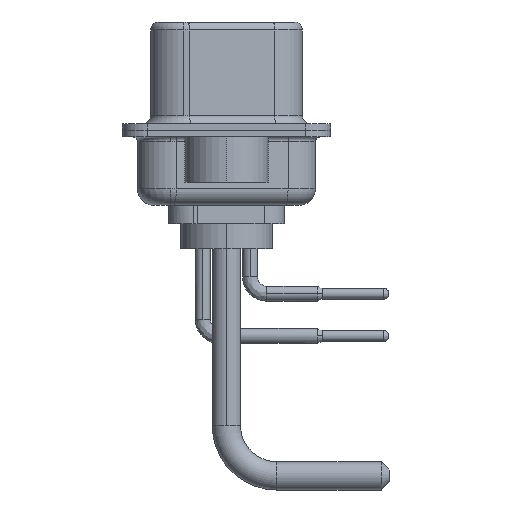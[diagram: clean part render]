
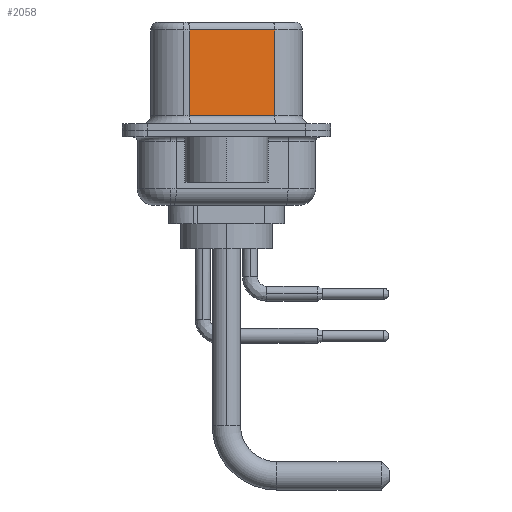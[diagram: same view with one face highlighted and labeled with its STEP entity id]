
A CAD part, left-side view. The second image highlights one B-rep face of the part: STEP entity #2058.
In plain terms, the highlighted planar face has unit normal (-0.985, -0.174, 0).
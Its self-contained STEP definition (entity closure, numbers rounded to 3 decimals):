
#1162 = ORIENTED_EDGE ( 'NONE', *, *, #23147, .F. ) ;
#2058 = ADVANCED_FACE ( 'NONE', ( #18580 ), #20807, .F. ) ;
#2570 = DIRECTION ( 'NONE',  ( 0.174, -0.985, 0. ) ) ;
#2748 = VERTEX_POINT ( 'NONE', #22221 ) ;
#3128 = CARTESIAN_POINT ( 'NONE',  ( 3.68, 2.203, 6.52 ) ) ;
#3800 = AXIS2_PLACEMENT_3D ( 'NONE', #7281, #7531, #9522 ) ;
#4761 = DIRECTION ( 'NONE',  ( 0., 0., -1. ) ) ;
#5580 = VECTOR ( 'NONE', #10281, 1000. ) ;
#5719 = CARTESIAN_POINT ( 'NONE',  ( 3.68, 2.203, 0.9 ) ) ;
#6299 = EDGE_CURVE ( 'NONE', #6349, #15088, #7669, .T. ) ;
#6349 = VERTEX_POINT ( 'NONE', #14748 ) ;
#6890 = VECTOR ( 'NONE', #4761, 1000. ) ;
#7281 = CARTESIAN_POINT ( 'NONE',  ( 4.58, -2.897, 6.52 ) ) ;
#7531 = DIRECTION ( 'NONE',  ( 0.985, 0.174, 0. ) ) ;
#7546 = DIRECTION ( 'NONE',  ( -0.174, 0.985, 0. ) ) ;
#7669 = LINE ( 'NONE', #16999, #15226 ) ;
#8403 = CARTESIAN_POINT ( 'NONE',  ( 4.58, -2.897, 0.9 ) ) ;
#8414 = EDGE_CURVE ( 'NONE', #15088, #20680, #16209, .T. ) ;
#8791 = CARTESIAN_POINT ( 'NONE',  ( 3.68, 2.203, 6.02 ) ) ;
#9522 = DIRECTION ( 'NONE',  ( -0.174, 0.985, 0. ) ) ;
#10281 = DIRECTION ( 'NONE',  ( 0., 0., -1. ) ) ;
#12036 = LINE ( 'NONE', #15764, #5580 ) ;
#12721 = VECTOR ( 'NONE', #2570, 1000. ) ;
#13962 = ORIENTED_EDGE ( 'NONE', *, *, #16571, .T. ) ;
#14748 = CARTESIAN_POINT ( 'NONE',  ( 4.58, -2.897, 6.02 ) ) ;
#15088 = VERTEX_POINT ( 'NONE', #8791 ) ;
#15226 = VECTOR ( 'NONE', #7546, 1000. ) ;
#15764 = CARTESIAN_POINT ( 'NONE',  ( 4.58, -2.897, 6.52 ) ) ;
#16209 = LINE ( 'NONE', #3128, #6890 ) ;
#16571 = EDGE_CURVE ( 'NONE', #20680, #2748, #19583, .T. ) ;
#16999 = CARTESIAN_POINT ( 'NONE',  ( 4.58, -2.897, 6.02 ) ) ;
#17086 = ORIENTED_EDGE ( 'NONE', *, *, #8414, .T. ) ;
#18117 = ORIENTED_EDGE ( 'NONE', *, *, #6299, .T. ) ;
#18580 = FACE_OUTER_BOUND ( 'NONE', #21335, .T. ) ;
#19583 = LINE ( 'NONE', #8403, #12721 ) ;
#20680 = VERTEX_POINT ( 'NONE', #5719 ) ;
#20807 = PLANE ( 'NONE',  #3800 ) ;
#21335 = EDGE_LOOP ( 'NONE', ( #1162, #18117, #17086, #13962 ) ) ;
#22221 = CARTESIAN_POINT ( 'NONE',  ( 4.58, -2.897, 0.9 ) ) ;
#23147 = EDGE_CURVE ( 'NONE', #6349, #2748, #12036, .T. ) ;
